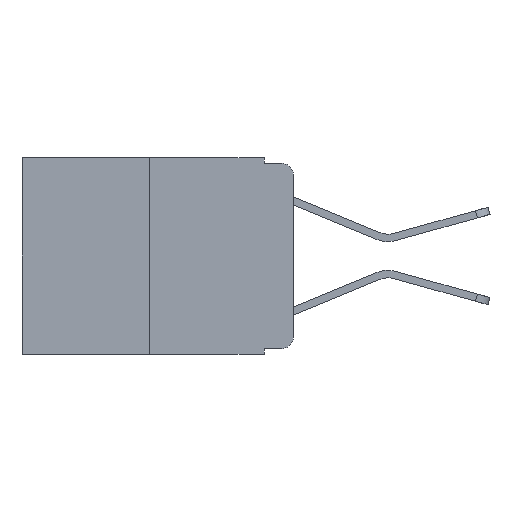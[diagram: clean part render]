
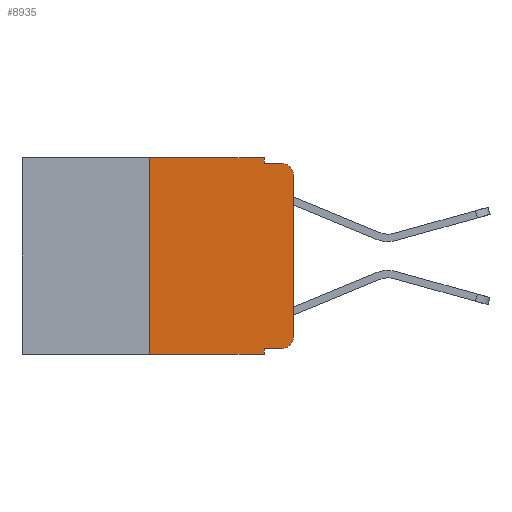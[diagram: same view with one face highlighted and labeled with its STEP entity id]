
A CAD part, left-side view. The second image highlights one B-rep face of the part: STEP entity #8935.
In plain terms, the highlighted planar face has unit normal (-1, 0, 0).
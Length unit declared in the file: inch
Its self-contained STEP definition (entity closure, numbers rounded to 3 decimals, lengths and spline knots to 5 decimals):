
#46 = CARTESIAN_POINT ( 'NONE',  ( 0., 0., -0.03 ) ) ;
#88 = VERTEX_POINT ( 'NONE', #4026 ) ;
#127 = VECTOR ( 'NONE', #10635, 39.37008 ) ;
#529 = DIRECTION ( 'NONE',  ( 1., 0., 0. ) ) ;
#792 = CARTESIAN_POINT ( 'NONE',  ( 0., 0.051, -0.333 ) ) ;
#1190 = DIRECTION ( 'NONE',  ( 0., -1., 0. ) ) ;
#1316 = VERTEX_POINT ( 'NONE', #10385 ) ;
#1647 = CIRCLE ( 'NONE', #10398, 0.02 ) ;
#1670 = CARTESIAN_POINT ( 'NONE',  ( 0., 0.051, -0.01 ) ) ;
#1993 = FACE_OUTER_BOUND ( 'NONE', #2758, .T. ) ;
#2000 = EDGE_CURVE ( 'NONE', #12113, #5845, #8836, .T. ) ;
#2056 = CARTESIAN_POINT ( 'NONE',  ( 0., 0.473, -0.343 ) ) ;
#2427 = DIRECTION ( 'NONE',  ( 0., 0., 1. ) ) ;
#2587 = VECTOR ( 'NONE', #6248, 39.37008 ) ;
#2718 = VERTEX_POINT ( 'NONE', #10023 ) ;
#2758 = EDGE_LOOP ( 'NONE', ( #4696, #4439, #5728, #4710, #4550, #3789, #4599, #3872, #4519, #4484 ) ) ;
#2928 = CARTESIAN_POINT ( 'NONE',  ( 0., 0.02, -0.03 ) ) ;
#3049 = EDGE_CURVE ( 'NONE', #4198, #1316, #3257, .T. ) ;
#3154 = CARTESIAN_POINT ( 'NONE',  ( 0., 0.25, 0. ) ) ;
#3257 = LINE ( 'NONE', #2056, #127 ) ;
#3340 = CIRCLE ( 'NONE', #10495, 0.02 ) ;
#3433 = VECTOR ( 'NONE', #7602, 39.37008 ) ;
#3789 = ORIENTED_EDGE ( 'NONE', *, *, #10872, .F. ) ;
#3872 = ORIENTED_EDGE ( 'NONE', *, *, #9662, .F. ) ;
#4026 = CARTESIAN_POINT ( 'NONE',  ( 0., 0.02, -0.01 ) ) ;
#4095 = DIRECTION ( 'NONE',  ( 0., 0., -1. ) ) ;
#4198 = VERTEX_POINT ( 'NONE', #6035 ) ;
#4311 = CARTESIAN_POINT ( 'NONE',  ( 0., 0.473, 0. ) ) ;
#4439 = ORIENTED_EDGE ( 'NONE', *, *, #13762, .T. ) ;
#4484 = ORIENTED_EDGE ( 'NONE', *, *, #6032, .T. ) ;
#4519 = ORIENTED_EDGE ( 'NONE', *, *, #8194, .T. ) ;
#4550 = ORIENTED_EDGE ( 'NONE', *, *, #2000, .F. ) ;
#4599 = ORIENTED_EDGE ( 'NONE', *, *, #3049, .T. ) ;
#4696 = ORIENTED_EDGE ( 'NONE', *, *, #11828, .T. ) ;
#4710 = ORIENTED_EDGE ( 'NONE', *, *, #12265, .F. ) ;
#4994 = VECTOR ( 'NONE', #2427, 39.37008 ) ;
#5201 = CARTESIAN_POINT ( 'NONE',  ( 0., 0.051, -0.333 ) ) ;
#5330 = LINE ( 'NONE', #8925, #4994 ) ;
#5517 = CARTESIAN_POINT ( 'NONE',  ( 0., 0.051, 0. ) ) ;
#5678 = DIRECTION ( 'NONE',  ( -1., 0., 0. ) ) ;
#5728 = ORIENTED_EDGE ( 'NONE', *, *, #12347, .F. ) ;
#5845 = VERTEX_POINT ( 'NONE', #13435 ) ;
#6032 = EDGE_CURVE ( 'NONE', #2718, #6573, #3340, .T. ) ;
#6035 = CARTESIAN_POINT ( 'NONE',  ( 0., 0.25, -0.343 ) ) ;
#6048 = LINE ( 'NONE', #5517, #3433 ) ;
#6248 = DIRECTION ( 'NONE',  ( 0., -1., 0. ) ) ;
#6573 = VERTEX_POINT ( 'NONE', #11660 ) ;
#6758 = VECTOR ( 'NONE', #1190, 39.37008 ) ;
#6970 = LINE ( 'NONE', #3154, #12039 ) ;
#7490 = DIRECTION ( 'NONE',  ( 0., 0., 1. ) ) ;
#7602 = DIRECTION ( 'NONE',  ( 0., 0., -1. ) ) ;
#7865 = CARTESIAN_POINT ( 'NONE',  ( 0., 0.051, -0.01 ) ) ;
#8085 = LINE ( 'NONE', #8783, #10471 ) ;
#8194 = EDGE_CURVE ( 'NONE', #12748, #2718, #8362, .T. ) ;
#8303 = DIRECTION ( 'NONE',  ( 0., 0., -1. ) ) ;
#8362 = LINE ( 'NONE', #5201, #2587 ) ;
#8506 = VECTOR ( 'NONE', #8512, 39.37008 ) ;
#8512 = DIRECTION ( 'NONE',  ( 0., -1., 0. ) ) ;
#8554 = VERTEX_POINT ( 'NONE', #46 ) ;
#8783 = CARTESIAN_POINT ( 'NONE',  ( 0., 0.051, 0. ) ) ;
#8836 = LINE ( 'NONE', #4311, #8506 ) ;
#8925 = CARTESIAN_POINT ( 'NONE',  ( 0., 0., 0. ) ) ;
#8935 = ADVANCED_FACE ( 'NONE', ( #1993 ), #12278, .F. ) ;
#9357 = CARTESIAN_POINT ( 'NONE',  ( 0., 0.25, 0. ) ) ;
#9662 = EDGE_CURVE ( 'NONE', #12748, #1316, #6048, .T. ) ;
#9821 = DIRECTION ( 'NONE',  ( 0., 0., -1. ) ) ;
#10023 = CARTESIAN_POINT ( 'NONE',  ( 0., 0.02, -0.333 ) ) ;
#10099 = VERTEX_POINT ( 'NONE', #1670 ) ;
#10377 = DIRECTION ( 'NONE',  ( -1., 0., 0. ) ) ;
#10385 = CARTESIAN_POINT ( 'NONE',  ( 0., 0.051, -0.343 ) ) ;
#10398 = AXIS2_PLACEMENT_3D ( 'NONE', #2928, #10377, #4095 ) ;
#10471 = VECTOR ( 'NONE', #9821, 39.37008 ) ;
#10495 = AXIS2_PLACEMENT_3D ( 'NONE', #11757, #5678, #12768 ) ;
#10635 = DIRECTION ( 'NONE',  ( 0., -1., 0. ) ) ;
#10872 = EDGE_CURVE ( 'NONE', #4198, #12113, #6970, .T. ) ;
#11660 = CARTESIAN_POINT ( 'NONE',  ( 0., 0., -0.313 ) ) ;
#11757 = CARTESIAN_POINT ( 'NONE',  ( 0., 0.02, -0.313 ) ) ;
#11828 = EDGE_CURVE ( 'NONE', #6573, #8554, #5330, .T. ) ;
#12039 = VECTOR ( 'NONE', #7490, 39.37008 ) ;
#12113 = VERTEX_POINT ( 'NONE', #9357 ) ;
#12265 = EDGE_CURVE ( 'NONE', #5845, #10099, #8085, .T. ) ;
#12278 = PLANE ( 'NONE',  #13328 ) ;
#12347 = EDGE_CURVE ( 'NONE', #10099, #88, #12457, .T. ) ;
#12457 = LINE ( 'NONE', #7865, #6758 ) ;
#12748 = VERTEX_POINT ( 'NONE', #792 ) ;
#12768 = DIRECTION ( 'NONE',  ( 0., 0., -1. ) ) ;
#13292 = CARTESIAN_POINT ( 'NONE',  ( 0., 0.473, 0. ) ) ;
#13328 = AXIS2_PLACEMENT_3D ( 'NONE', #13292, #529, #8303 ) ;
#13435 = CARTESIAN_POINT ( 'NONE',  ( 0., 0.051, 0. ) ) ;
#13762 = EDGE_CURVE ( 'NONE', #8554, #88, #1647, .T. ) ;
